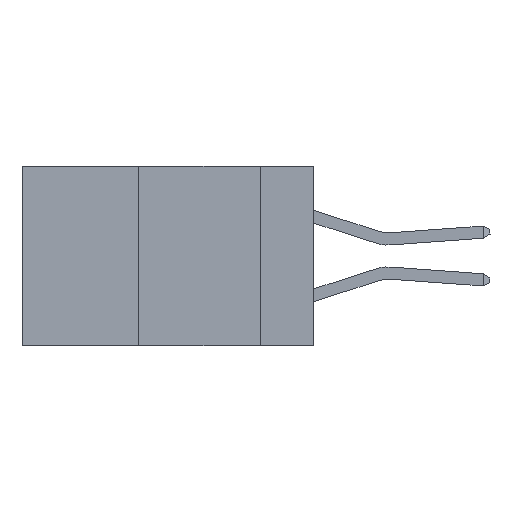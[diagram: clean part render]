
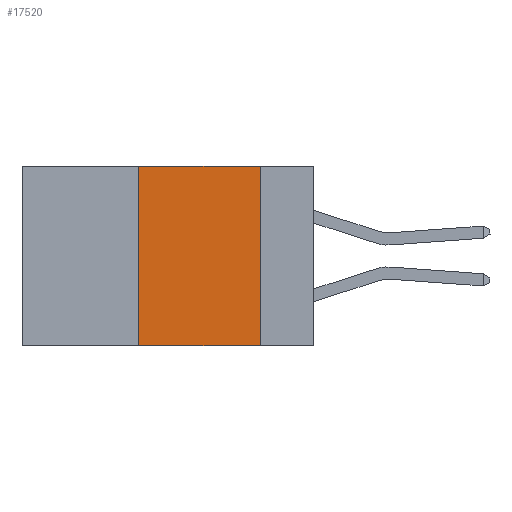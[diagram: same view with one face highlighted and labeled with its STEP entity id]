
A CAD part, left-side view. The second image highlights one B-rep face of the part: STEP entity #17520.
In plain terms, the highlighted planar face has unit normal (-1, 0, 0).
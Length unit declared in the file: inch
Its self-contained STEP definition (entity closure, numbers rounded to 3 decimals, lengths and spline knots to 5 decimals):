
#396 = CARTESIAN_POINT ( 'NONE',  ( 0., 0.36, -0.37 ) ) ;
#871 = FACE_OUTER_BOUND ( 'NONE', #22031, .T. ) ;
#1898 = ORIENTED_EDGE ( 'NONE', *, *, #4296, .F. ) ;
#2894 = CARTESIAN_POINT ( 'NONE',  ( 0., 0.36, 0. ) ) ;
#3648 = EDGE_CURVE ( 'NONE', #9296, #4824, #12951, .T. ) ;
#4106 = ORIENTED_EDGE ( 'NONE', *, *, #18379, .F. ) ;
#4296 = EDGE_CURVE ( 'NONE', #4824, #19347, #26217, .T. ) ;
#4362 = CARTESIAN_POINT ( 'NONE',  ( 0., 0.11, 0. ) ) ;
#4824 = VERTEX_POINT ( 'NONE', #2894 ) ;
#5100 = DIRECTION ( 'NONE',  ( 0., -1., 0. ) ) ;
#5652 = VECTOR ( 'NONE', #5100, 39.37008 ) ;
#6850 = VECTOR ( 'NONE', #25505, 39.37008 ) ;
#7287 = VECTOR ( 'NONE', #22190, 39.37008 ) ;
#7847 = VECTOR ( 'NONE', #10959, 39.37008 ) ;
#8849 = EDGE_CURVE ( 'NONE', #9296, #15844, #19127, .T. ) ;
#9296 = VERTEX_POINT ( 'NONE', #396 ) ;
#10290 = DIRECTION ( 'NONE',  ( 0., 0., -1. ) ) ;
#10298 = CARTESIAN_POINT ( 'NONE',  ( 0., 0.6, 0. ) ) ;
#10959 = DIRECTION ( 'NONE',  ( 0., -1., 0. ) ) ;
#11343 = CARTESIAN_POINT ( 'NONE',  ( 0., 0.6, -0.37 ) ) ;
#12951 = LINE ( 'NONE', #26285, #7287 ) ;
#14472 = PLANE ( 'NONE',  #17509 ) ;
#14606 = CARTESIAN_POINT ( 'NONE',  ( 0., 0.11, 0. ) ) ;
#15844 = VERTEX_POINT ( 'NONE', #17135 ) ;
#17135 = CARTESIAN_POINT ( 'NONE',  ( 0., 0.11, -0.37 ) ) ;
#17509 = AXIS2_PLACEMENT_3D ( 'NONE', #18982, #23249, #10290 ) ;
#17520 = ADVANCED_FACE ( 'NONE', ( #871 ), #14472, .F. ) ;
#18379 = EDGE_CURVE ( 'NONE', #19347, #15844, #21087, .T. ) ;
#18982 = CARTESIAN_POINT ( 'NONE',  ( 0., 0.6, 0. ) ) ;
#19127 = LINE ( 'NONE', #11343, #7847 ) ;
#19347 = VERTEX_POINT ( 'NONE', #14606 ) ;
#21087 = LINE ( 'NONE', #4362, #6850 ) ;
#22031 = EDGE_LOOP ( 'NONE', ( #4106, #1898, #26136, #22835 ) ) ;
#22190 = DIRECTION ( 'NONE',  ( 0., 0., 1. ) ) ;
#22835 = ORIENTED_EDGE ( 'NONE', *, *, #8849, .T. ) ;
#23249 = DIRECTION ( 'NONE',  ( 1., 0., 0. ) ) ;
#25505 = DIRECTION ( 'NONE',  ( 0., 0., -1. ) ) ;
#26136 = ORIENTED_EDGE ( 'NONE', *, *, #3648, .F. ) ;
#26217 = LINE ( 'NONE', #10298, #5652 ) ;
#26285 = CARTESIAN_POINT ( 'NONE',  ( 0., 0.36, 0. ) ) ;
